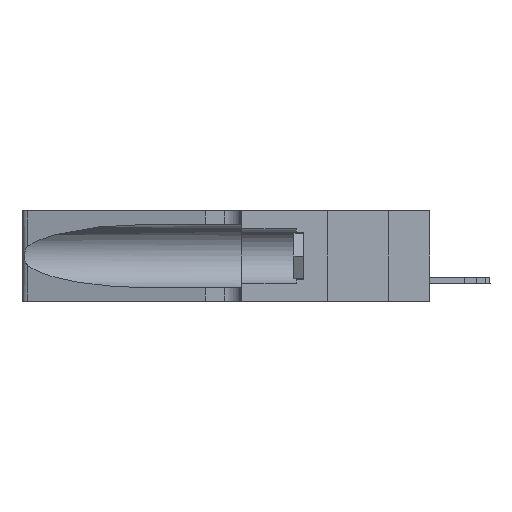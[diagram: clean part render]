
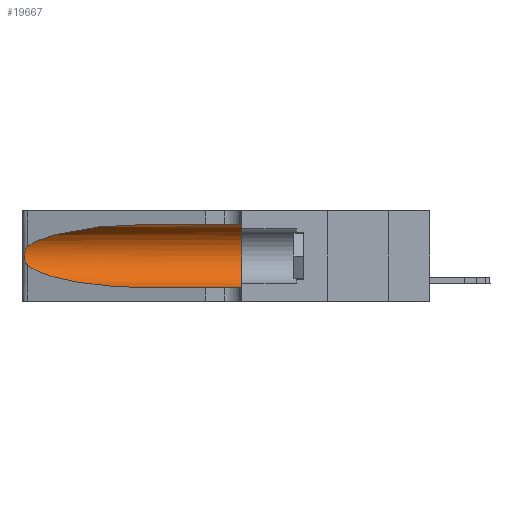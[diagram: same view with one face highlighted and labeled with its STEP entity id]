
A CAD part, left-side view. The second image highlights one B-rep face of the part: STEP entity #19667.
In plain terms, the highlighted cylindrical face has radius 3.308 mm (diameter 6.617 mm), a partial arc.
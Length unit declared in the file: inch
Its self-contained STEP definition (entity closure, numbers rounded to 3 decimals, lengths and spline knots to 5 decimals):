
#375 = EDGE_LOOP ( 'NONE', ( #20568, #6144, #14852, #28886, #27063, #30775 ) ) ;
#1237 = CARTESIAN_POINT ( 'NONE',  ( 0.1305, 0.35, 0.05475 ) ) ;
#1303 =( BOUNDED_CURVE ( )  B_SPLINE_CURVE ( 3, ( #18651, #16542, #14116, #23513 ),
 .UNSPECIFIED., .F., .F. ) 
 B_SPLINE_CURVE_WITH_KNOTS ( ( 4, 4 ),
 ( 3.44316, 4.71239 ),
 .UNSPECIFIED. ) 
 CURVE ( )  GEOMETRIC_REPRESENTATION_ITEM ( )  RATIONAL_B_SPLINE_CURVE ( ( 1., 0.87, 0.87, 1. ) ) 
 REPRESENTATION_ITEM ( '' )  );
#1312 = VERTEX_POINT ( 'NONE', #16964 ) ;
#1907 = AXIS2_PLACEMENT_3D ( 'NONE', #22332, #27423, #17887 ) ;
#1913 = CARTESIAN_POINT ( 'NONE',  ( 0.25639, 1.23184, 0.21858 ) ) ;
#2062 = CARTESIAN_POINT ( 'NONE',  ( 0.1305, 0.72297, 0.31525 ) ) ;
#2211 = AXIS2_PLACEMENT_3D ( 'NONE', #13779, #26089, #16408 ) ;
#2335 = CIRCLE ( 'NONE', #1907, 0.13025 ) ;
#3211 = VERTEX_POINT ( 'NONE', #2062 ) ;
#4435 = CARTESIAN_POINT ( 'NONE',  ( 0.25555, 1.22994, 0.2215 ) ) ;
#5093 = DIRECTION ( 'NONE',  ( 0., -1., 0. ) ) ;
#5331 = CARTESIAN_POINT ( 'NONE',  ( 0.25487, 1.22718, 0.14631 ) ) ;
#6144 = ORIENTED_EDGE ( 'NONE', *, *, #25336, .T. ) ;
#6513 = CARTESIAN_POINT ( 'NONE',  ( 0.26075, 1.23896, 0.19203 ) ) ;
#6615 = CARTESIAN_POINT ( 'NONE',  ( 0.25856, 1.23593, 0.16098 ) ) ;
#6844 = CARTESIAN_POINT ( 'NONE',  ( 0.25789, 1.23486, 0.15765 ) ) ;
#6874 = CYLINDRICAL_SURFACE ( 'NONE', #2211, 0.13025 ) ;
#6927 = VECTOR ( 'NONE', #19074, 39.37008 ) ;
#8460 = VERTEX_POINT ( 'NONE', #1237 ) ;
#9918 = CARTESIAN_POINT ( 'NONE',  ( 0.2373, 1.15595, 0.28018 ) ) ;
#10250 = CARTESIAN_POINT ( 'NONE',  ( 0.1305, 0.35, 0.31525 ) ) ;
#10996 = B_SPLINE_CURVE_WITH_KNOTS ( 'NONE', 3,
 ( #28472, #4435, #1913, #31109, #21283, #28582, #6513, #18731, #26171, #6615, #6844, #23692, #18845, #28689 ),
 .UNSPECIFIED., .F., .F.,
 ( 4, 2, 2, 2, 2, 2, 4 ),
 ( 0., 0.00027, 0.00053, 0.00107, 0.0016, 0.00187, 0.00214 ),
 .UNSPECIFIED. ) ;
#12334 = CARTESIAN_POINT ( 'NONE',  ( 0.1305, 1.61858, 0.05475 ) ) ;
#13427 = LINE ( 'NONE', #16271, #6927 ) ;
#13434 = EDGE_CURVE ( 'NONE', #26658, #8460, #2335, .T. ) ;
#13779 = CARTESIAN_POINT ( 'NONE',  ( 0.1305, 1.61858, 0.185 ) ) ;
#14116 = CARTESIAN_POINT ( 'NONE',  ( 0.18966, 0.96281, 0.05475 ) ) ;
#14852 = ORIENTED_EDGE ( 'NONE', *, *, #21577, .T. ) ;
#16271 = CARTESIAN_POINT ( 'NONE',  ( 0.1305, 1.61858, 0.31525 ) ) ;
#16408 = DIRECTION ( 'NONE',  ( 0., 0., -1. ) ) ;
#16542 = CARTESIAN_POINT ( 'NONE',  ( 0.2373, 1.15595, 0.08982 ) ) ;
#16657 =( BOUNDED_CURVE ( )  B_SPLINE_CURVE ( 3, ( #30797, #23824, #9918, #29613 ),
 .UNSPECIFIED., .F., .F. ) 
 B_SPLINE_CURVE_WITH_KNOTS ( ( 4, 4 ),
 ( 1.5708, 2.84003 ),
 .UNSPECIFIED. ) 
 CURVE ( )  GEOMETRIC_REPRESENTATION_ITEM ( )  RATIONAL_B_SPLINE_CURVE ( ( 1., 0.87, 0.87, 1. ) ) 
 REPRESENTATION_ITEM ( '' )  );
#16964 = CARTESIAN_POINT ( 'NONE',  ( 0.1305, 0.72297, 0.05475 ) ) ;
#17887 = DIRECTION ( 'NONE',  ( 0., 0., 1. ) ) ;
#18651 = CARTESIAN_POINT ( 'NONE',  ( 0.25487, 1.22718, 0.14631 ) ) ;
#18731 = CARTESIAN_POINT ( 'NONE',  ( 0.26075, 1.23896, 0.178 ) ) ;
#18845 = CARTESIAN_POINT ( 'NONE',  ( 0.25555, 1.22993, 0.14849 ) ) ;
#19074 = DIRECTION ( 'NONE',  ( 0., -1., 0. ) ) ;
#19098 = EDGE_CURVE ( 'NONE', #3211, #26658, #13427, .T. ) ;
#19667 = ADVANCED_FACE ( 'NONE', ( #21700 ), #6874, .F. ) ;
#20568 = ORIENTED_EDGE ( 'NONE', *, *, #22979, .T. ) ;
#20663 = VERTEX_POINT ( 'NONE', #24765 ) ;
#21283 = CARTESIAN_POINT ( 'NONE',  ( 0.25854, 1.2359, 0.20912 ) ) ;
#21577 = EDGE_CURVE ( 'NONE', #24706, #1312, #1303, .T. ) ;
#21700 = FACE_OUTER_BOUND ( 'NONE', #375, .T. ) ;
#22332 = CARTESIAN_POINT ( 'NONE',  ( 0.1305, 0.35, 0.185 ) ) ;
#22400 = VECTOR ( 'NONE', #5093, 39.37008 ) ;
#22979 = EDGE_CURVE ( 'NONE', #3211, #20663, #16657, .T. ) ;
#23513 = CARTESIAN_POINT ( 'NONE',  ( 0.1305, 0.72297, 0.05475 ) ) ;
#23692 = CARTESIAN_POINT ( 'NONE',  ( 0.25639, 1.23186, 0.15144 ) ) ;
#23824 = CARTESIAN_POINT ( 'NONE',  ( 0.18966, 0.96281, 0.31525 ) ) ;
#24706 = VERTEX_POINT ( 'NONE', #5331 ) ;
#24765 = CARTESIAN_POINT ( 'NONE',  ( 0.25487, 1.22718, 0.22369 ) ) ;
#25336 = EDGE_CURVE ( 'NONE', #20663, #24706, #10996, .T. ) ;
#26089 = DIRECTION ( 'NONE',  ( 0., -1., 0. ) ) ;
#26171 = CARTESIAN_POINT ( 'NONE',  ( 0.26017, 1.23833, 0.17102 ) ) ;
#26252 = LINE ( 'NONE', #12334, #22400 ) ;
#26658 = VERTEX_POINT ( 'NONE', #10250 ) ;
#27063 = ORIENTED_EDGE ( 'NONE', *, *, #13434, .F. ) ;
#27423 = DIRECTION ( 'NONE',  ( 0., 1., 0. ) ) ;
#27760 = EDGE_CURVE ( 'NONE', #1312, #8460, #26252, .T. ) ;
#28472 = CARTESIAN_POINT ( 'NONE',  ( 0.25487, 1.22718, 0.22369 ) ) ;
#28582 = CARTESIAN_POINT ( 'NONE',  ( 0.26018, 1.23835, 0.19895 ) ) ;
#28689 = CARTESIAN_POINT ( 'NONE',  ( 0.25487, 1.22718, 0.14631 ) ) ;
#28886 = ORIENTED_EDGE ( 'NONE', *, *, #27760, .T. ) ;
#29613 = CARTESIAN_POINT ( 'NONE',  ( 0.25487, 1.22718, 0.22369 ) ) ;
#30775 = ORIENTED_EDGE ( 'NONE', *, *, #19098, .F. ) ;
#30797 = CARTESIAN_POINT ( 'NONE',  ( 0.1305, 0.72297, 0.31525 ) ) ;
#31109 = CARTESIAN_POINT ( 'NONE',  ( 0.25787, 1.23484, 0.2124 ) ) ;
